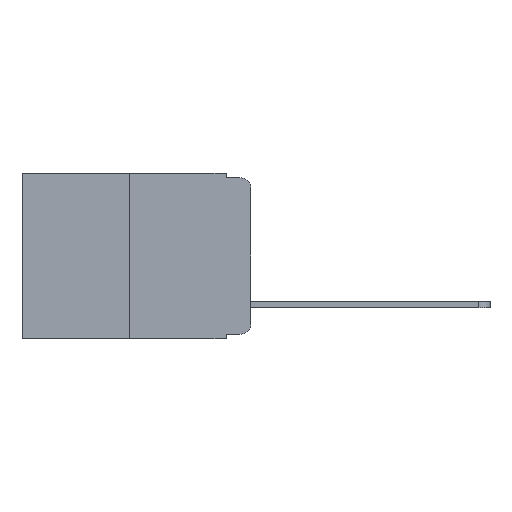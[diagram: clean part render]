
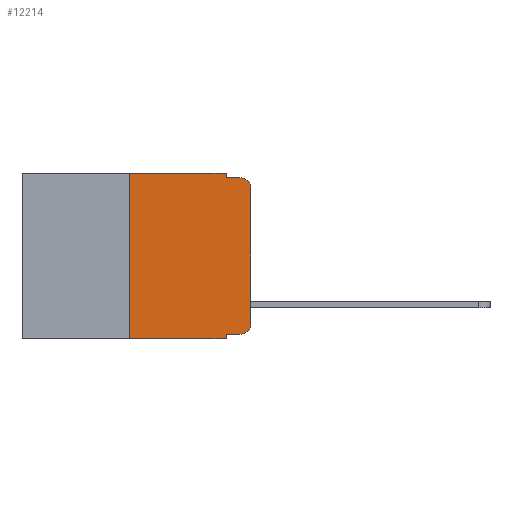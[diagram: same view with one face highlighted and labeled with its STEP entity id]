
A CAD part, left-side view. The second image highlights one B-rep face of the part: STEP entity #12214.
In plain terms, the highlighted planar face has unit normal (-1, 0, 0).
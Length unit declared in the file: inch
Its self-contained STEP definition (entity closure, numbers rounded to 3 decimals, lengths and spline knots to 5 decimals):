
#185 = AXIS2_PLACEMENT_3D ( 'NONE', #7776, #20780, #5896 ) ;
#364 = PLANE ( 'NONE',  #185 ) ;
#1027 = CARTESIAN_POINT ( 'NONE',  ( 0., 0.02, -0.333 ) ) ;
#1087 = VECTOR ( 'NONE', #10434, 39.37008 ) ;
#1326 = DIRECTION ( 'NONE',  ( 0., 0., 1. ) ) ;
#1775 = ORIENTED_EDGE ( 'NONE', *, *, #21943, .T. ) ;
#2159 = ORIENTED_EDGE ( 'NONE', *, *, #8371, .T. ) ;
#2204 = EDGE_CURVE ( 'NONE', #12095, #9939, #10740, .T. ) ;
#2236 = LINE ( 'NONE', #23371, #13629 ) ;
#2302 = VERTEX_POINT ( 'NONE', #18340 ) ;
#2410 = EDGE_CURVE ( 'NONE', #2302, #9404, #5449, .T. ) ;
#3213 = DIRECTION ( 'NONE',  ( 0., 0., -1. ) ) ;
#3364 = EDGE_CURVE ( 'NONE', #20492, #9939, #6912, .T. ) ;
#4804 = LINE ( 'NONE', #10045, #16227 ) ;
#5116 = ORIENTED_EDGE ( 'NONE', *, *, #3364, .F. ) ;
#5294 = LINE ( 'NONE', #14159, #13799 ) ;
#5302 = DIRECTION ( 'NONE',  ( -1., 0., 0. ) ) ;
#5438 = EDGE_CURVE ( 'NONE', #6168, #12095, #5294, .T. ) ;
#5449 = LINE ( 'NONE', #8729, #1087 ) ;
#5451 = DIRECTION ( 'NONE',  ( 0., 0., -1. ) ) ;
#5896 = DIRECTION ( 'NONE',  ( 0., 0., -1. ) ) ;
#6168 = VERTEX_POINT ( 'NONE', #12827 ) ;
#6332 = DIRECTION ( 'NONE',  ( 0., 0., -1. ) ) ;
#6372 = VERTEX_POINT ( 'NONE', #9887 ) ;
#6754 = CARTESIAN_POINT ( 'NONE',  ( 0., 0.051, -0.01 ) ) ;
#6912 = LINE ( 'NONE', #6754, #18335 ) ;
#7149 = EDGE_CURVE ( 'NONE', #6372, #2302, #18118, .T. ) ;
#7776 = CARTESIAN_POINT ( 'NONE',  ( 0., 0.473, 0. ) ) ;
#8371 = EDGE_CURVE ( 'NONE', #15598, #6168, #13315, .T. ) ;
#8519 = DIRECTION ( 'NONE',  ( 0., -1., 0. ) ) ;
#8598 = DIRECTION ( 'NONE',  ( 0., 0., 1. ) ) ;
#8614 = EDGE_CURVE ( 'NONE', #17019, #17545, #4804, .T. ) ;
#8729 = CARTESIAN_POINT ( 'NONE',  ( 0., 0.473, 0. ) ) ;
#8777 = CARTESIAN_POINT ( 'NONE',  ( 0., 0.051, 0. ) ) ;
#8997 = ORIENTED_EDGE ( 'NONE', *, *, #8614, .F. ) ;
#9193 = CARTESIAN_POINT ( 'NONE',  ( 0., 0., -0.03 ) ) ;
#9235 = CARTESIAN_POINT ( 'NONE',  ( 0., 0.02, -0.313 ) ) ;
#9404 = VERTEX_POINT ( 'NONE', #12288 ) ;
#9485 = DIRECTION ( 'NONE',  ( -1., 0., 0. ) ) ;
#9666 = LINE ( 'NONE', #23241, #15214 ) ;
#9887 = CARTESIAN_POINT ( 'NONE',  ( 0., 0.25, -0.343 ) ) ;
#9939 = VERTEX_POINT ( 'NONE', #10153 ) ;
#10045 = CARTESIAN_POINT ( 'NONE',  ( 0., 0.051, 0. ) ) ;
#10153 = CARTESIAN_POINT ( 'NONE',  ( 0., 0.02, -0.01 ) ) ;
#10434 = DIRECTION ( 'NONE',  ( 0., -1., 0. ) ) ;
#10740 = CIRCLE ( 'NONE', #21460, 0.02 ) ;
#11240 = CARTESIAN_POINT ( 'NONE',  ( 0., 0.051, -0.333 ) ) ;
#11337 = CARTESIAN_POINT ( 'NONE',  ( 0., 0.051, -0.01 ) ) ;
#12095 = VERTEX_POINT ( 'NONE', #9193 ) ;
#12214 = ADVANCED_FACE ( 'NONE', ( #13395 ), #364, .F. ) ;
#12288 = CARTESIAN_POINT ( 'NONE',  ( 0., 0.051, 0. ) ) ;
#12804 = VECTOR ( 'NONE', #3213, 39.37008 ) ;
#12827 = CARTESIAN_POINT ( 'NONE',  ( 0., 0., -0.313 ) ) ;
#13315 = CIRCLE ( 'NONE', #15023, 0.02 ) ;
#13395 = FACE_OUTER_BOUND ( 'NONE', #15478, .T. ) ;
#13629 = VECTOR ( 'NONE', #23460, 39.37008 ) ;
#13799 = VECTOR ( 'NONE', #1326, 39.37008 ) ;
#14159 = CARTESIAN_POINT ( 'NONE',  ( 0., 0., 0. ) ) ;
#14482 = ORIENTED_EDGE ( 'NONE', *, *, #7149, .F. ) ;
#15023 = AXIS2_PLACEMENT_3D ( 'NONE', #9235, #9485, #5451 ) ;
#15214 = VECTOR ( 'NONE', #8519, 39.37008 ) ;
#15435 = ORIENTED_EDGE ( 'NONE', *, *, #2410, .F. ) ;
#15478 = EDGE_LOOP ( 'NONE', ( #18254, #22534, #5116, #18473, #15435, #14482, #1775, #8997, #22348, #2159 ) ) ;
#15480 = VECTOR ( 'NONE', #8598, 39.37008 ) ;
#15598 = VERTEX_POINT ( 'NONE', #1027 ) ;
#15926 = DIRECTION ( 'NONE',  ( 0., -1., 0. ) ) ;
#16227 = VECTOR ( 'NONE', #6332, 39.37008 ) ;
#16518 = CARTESIAN_POINT ( 'NONE',  ( 0., 0.02, -0.03 ) ) ;
#17019 = VERTEX_POINT ( 'NONE', #11240 ) ;
#17545 = VERTEX_POINT ( 'NONE', #20036 ) ;
#18118 = LINE ( 'NONE', #19963, #15480 ) ;
#18254 = ORIENTED_EDGE ( 'NONE', *, *, #5438, .T. ) ;
#18335 = VECTOR ( 'NONE', #15926, 39.37008 ) ;
#18340 = CARTESIAN_POINT ( 'NONE',  ( 0., 0.25, 0. ) ) ;
#18473 = ORIENTED_EDGE ( 'NONE', *, *, #20906, .F. ) ;
#18962 = LINE ( 'NONE', #8777, #12804 ) ;
#19201 = EDGE_CURVE ( 'NONE', #17019, #15598, #9666, .T. ) ;
#19963 = CARTESIAN_POINT ( 'NONE',  ( 0., 0.25, 0. ) ) ;
#20036 = CARTESIAN_POINT ( 'NONE',  ( 0., 0.051, -0.343 ) ) ;
#20492 = VERTEX_POINT ( 'NONE', #11337 ) ;
#20780 = DIRECTION ( 'NONE',  ( 1., 0., 0. ) ) ;
#20906 = EDGE_CURVE ( 'NONE', #9404, #20492, #18962, .T. ) ;
#21460 = AXIS2_PLACEMENT_3D ( 'NONE', #16518, #5302, #24047 ) ;
#21943 = EDGE_CURVE ( 'NONE', #6372, #17545, #2236, .T. ) ;
#22348 = ORIENTED_EDGE ( 'NONE', *, *, #19201, .T. ) ;
#22534 = ORIENTED_EDGE ( 'NONE', *, *, #2204, .T. ) ;
#23241 = CARTESIAN_POINT ( 'NONE',  ( 0., 0.051, -0.333 ) ) ;
#23371 = CARTESIAN_POINT ( 'NONE',  ( 0., 0.473, -0.343 ) ) ;
#23460 = DIRECTION ( 'NONE',  ( 0., -1., 0. ) ) ;
#24047 = DIRECTION ( 'NONE',  ( 0., 0., -1. ) ) ;
